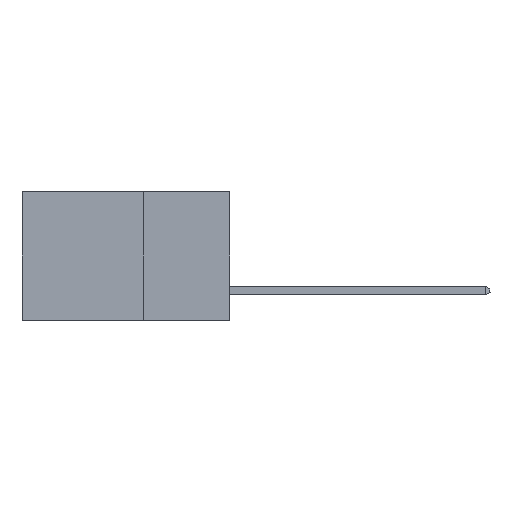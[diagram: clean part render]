
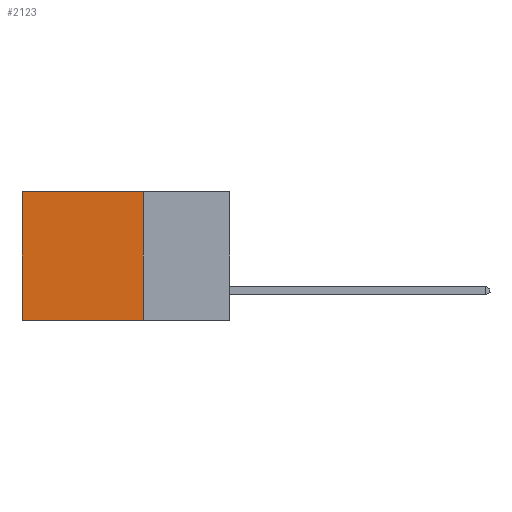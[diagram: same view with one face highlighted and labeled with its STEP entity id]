
A CAD part, left-side view. The second image highlights one B-rep face of the part: STEP entity #2123.
In plain terms, the highlighted planar face has unit normal (-1, 0, 0).
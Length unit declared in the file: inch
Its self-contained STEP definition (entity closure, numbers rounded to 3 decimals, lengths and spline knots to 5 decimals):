
#227 = VERTEX_POINT ( 'NONE', #13529 ) ;
#275 = LINE ( 'NONE', #10822, #3362 ) ;
#476 = VECTOR ( 'NONE', #9060, 39.37008 ) ;
#612 = EDGE_CURVE ( 'NONE', #227, #13075, #11300, .T. ) ;
#1017 = CARTESIAN_POINT ( 'NONE',  ( 0.298, 0.25, 0. ) ) ;
#1254 = CARTESIAN_POINT ( 'NONE',  ( 0.298, 0.6, 0. ) ) ;
#2123 = ADVANCED_FACE ( 'NONE', ( #15581 ), #12813, .F. ) ;
#2912 = DIRECTION ( 'NONE',  ( 0., 1., 0. ) ) ;
#2987 = VERTEX_POINT ( 'NONE', #3153 ) ;
#3153 = CARTESIAN_POINT ( 'NONE',  ( 0.298, 0.25, -0.37 ) ) ;
#3362 = VECTOR ( 'NONE', #2912, 39.37008 ) ;
#3586 = ORIENTED_EDGE ( 'NONE', *, *, #14280, .F. ) ;
#3631 = DIRECTION ( 'NONE',  ( 0., 0., -1. ) ) ;
#3803 = VERTEX_POINT ( 'NONE', #8411 ) ;
#4557 = LINE ( 'NONE', #1017, #9720 ) ;
#4898 = CARTESIAN_POINT ( 'NONE',  ( 0.298, 0.6, -0.37 ) ) ;
#5258 = DIRECTION ( 'NONE',  ( 0., 0., -1. ) ) ;
#5617 = EDGE_CURVE ( 'NONE', #2987, #13075, #275, .T. ) ;
#5984 = ORIENTED_EDGE ( 'NONE', *, *, #5617, .F. ) ;
#6260 = LINE ( 'NONE', #6407, #476 ) ;
#6336 = CARTESIAN_POINT ( 'NONE',  ( 0.298, 0.25, 0. ) ) ;
#6407 = CARTESIAN_POINT ( 'NONE',  ( 0.298, 0.25, 0. ) ) ;
#7564 = AXIS2_PLACEMENT_3D ( 'NONE', #6336, #10304, #3631 ) ;
#8411 = CARTESIAN_POINT ( 'NONE',  ( 0.298, 0.25, 0. ) ) ;
#8730 = EDGE_LOOP ( 'NONE', ( #15922, #5984, #3586, #16255 ) ) ;
#9060 = DIRECTION ( 'NONE',  ( 0., 1., 0. ) ) ;
#9720 = VECTOR ( 'NONE', #12982, 39.37008 ) ;
#10304 = DIRECTION ( 'NONE',  ( 1., 0., 0. ) ) ;
#10822 = CARTESIAN_POINT ( 'NONE',  ( 0.298, 0.25, -0.37 ) ) ;
#11300 = LINE ( 'NONE', #1254, #12148 ) ;
#12148 = VECTOR ( 'NONE', #5258, 39.37008 ) ;
#12813 = PLANE ( 'NONE',  #7564 ) ;
#12856 = EDGE_CURVE ( 'NONE', #3803, #227, #6260, .T. ) ;
#12982 = DIRECTION ( 'NONE',  ( 0., 0., -1. ) ) ;
#13075 = VERTEX_POINT ( 'NONE', #4898 ) ;
#13529 = CARTESIAN_POINT ( 'NONE',  ( 0.298, 0.6, 0. ) ) ;
#14280 = EDGE_CURVE ( 'NONE', #3803, #2987, #4557, .T. ) ;
#15581 = FACE_OUTER_BOUND ( 'NONE', #8730, .T. ) ;
#15922 = ORIENTED_EDGE ( 'NONE', *, *, #612, .T. ) ;
#16255 = ORIENTED_EDGE ( 'NONE', *, *, #12856, .T. ) ;
